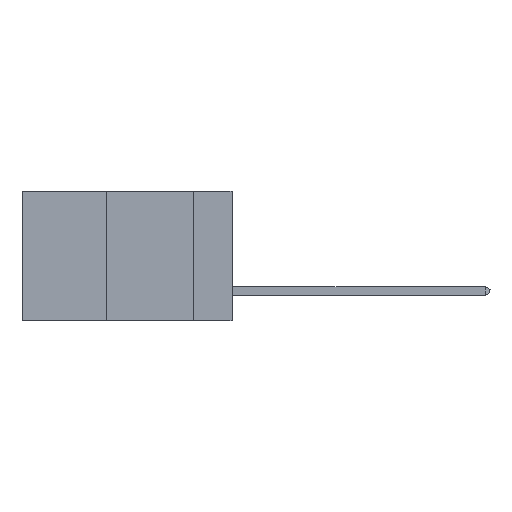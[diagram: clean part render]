
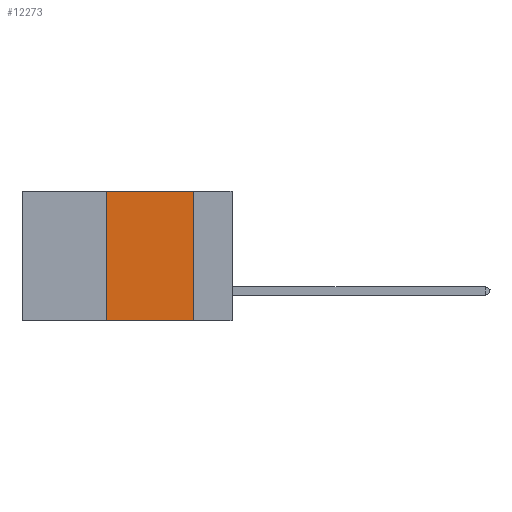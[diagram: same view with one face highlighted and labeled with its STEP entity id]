
A CAD part, left-side view. The second image highlights one B-rep face of the part: STEP entity #12273.
In plain terms, the highlighted planar face has unit normal (-1, 0, 0).
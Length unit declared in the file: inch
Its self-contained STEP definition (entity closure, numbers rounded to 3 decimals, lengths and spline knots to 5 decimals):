
#2088 = CARTESIAN_POINT ( 'NONE',  ( 0., 0.36, 0. ) ) ;
#2406 = CARTESIAN_POINT ( 'NONE',  ( 0., 0.11, 0. ) ) ;
#2826 = LINE ( 'NONE', #8075, #12192 ) ;
#2883 = CARTESIAN_POINT ( 'NONE',  ( 0., 0.36, -0.37 ) ) ;
#3350 = AXIS2_PLACEMENT_3D ( 'NONE', #14210, #4882, #6846 ) ;
#4254 = FACE_OUTER_BOUND ( 'NONE', #7040, .T. ) ;
#4423 = DIRECTION ( 'NONE',  ( 0., -1., 0. ) ) ;
#4634 = PLANE ( 'NONE',  #3350 ) ;
#4882 = DIRECTION ( 'NONE',  ( 1., 0., 0. ) ) ;
#5094 = VERTEX_POINT ( 'NONE', #2406 ) ;
#6419 = EDGE_CURVE ( 'NONE', #7656, #5094, #20773, .T. ) ;
#6846 = DIRECTION ( 'NONE',  ( 0., 0., -1. ) ) ;
#7040 = EDGE_LOOP ( 'NONE', ( #10414, #22528, #15025, #13540 ) ) ;
#7656 = VERTEX_POINT ( 'NONE', #2088 ) ;
#8075 = CARTESIAN_POINT ( 'NONE',  ( 0., 0.36, 0. ) ) ;
#8373 = VECTOR ( 'NONE', #12340, 39.37008 ) ;
#10414 = ORIENTED_EDGE ( 'NONE', *, *, #13479, .F. ) ;
#11265 = VECTOR ( 'NONE', #17120, 39.37008 ) ;
#11560 = LINE ( 'NONE', #23374, #8373 ) ;
#11831 = VERTEX_POINT ( 'NONE', #2883 ) ;
#12123 = VECTOR ( 'NONE', #4423, 39.37008 ) ;
#12192 = VECTOR ( 'NONE', #17790, 39.37008 ) ;
#12273 = ADVANCED_FACE ( 'NONE', ( #4254 ), #4634, .F. ) ;
#12340 = DIRECTION ( 'NONE',  ( 0., -1., 0. ) ) ;
#12576 = EDGE_CURVE ( 'NONE', #11831, #18105, #11560, .T. ) ;
#13258 = CARTESIAN_POINT ( 'NONE',  ( 0., 0.6, 0. ) ) ;
#13479 = EDGE_CURVE ( 'NONE', #5094, #18105, #21073, .T. ) ;
#13540 = ORIENTED_EDGE ( 'NONE', *, *, #12576, .T. ) ;
#14210 = CARTESIAN_POINT ( 'NONE',  ( 0., 0.6, 0. ) ) ;
#15025 = ORIENTED_EDGE ( 'NONE', *, *, #21597, .F. ) ;
#17120 = DIRECTION ( 'NONE',  ( 0., 0., -1. ) ) ;
#17790 = DIRECTION ( 'NONE',  ( 0., 0., 1. ) ) ;
#17901 = CARTESIAN_POINT ( 'NONE',  ( 0., 0.11, -0.37 ) ) ;
#18105 = VERTEX_POINT ( 'NONE', #17901 ) ;
#20773 = LINE ( 'NONE', #13258, #12123 ) ;
#21073 = LINE ( 'NONE', #22276, #11265 ) ;
#21597 = EDGE_CURVE ( 'NONE', #11831, #7656, #2826, .T. ) ;
#22276 = CARTESIAN_POINT ( 'NONE',  ( 0., 0.11, 0. ) ) ;
#22528 = ORIENTED_EDGE ( 'NONE', *, *, #6419, .F. ) ;
#23374 = CARTESIAN_POINT ( 'NONE',  ( 0., 0.6, -0.37 ) ) ;
